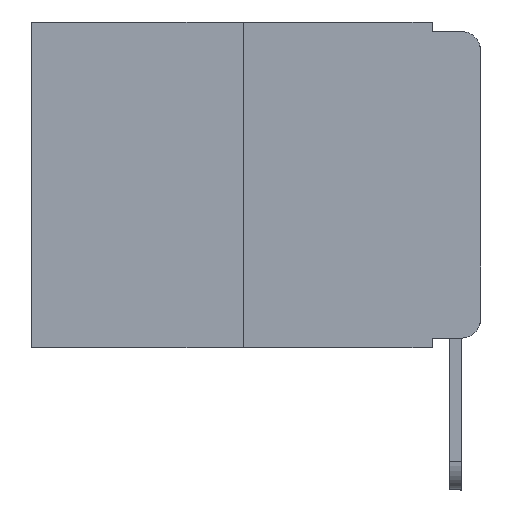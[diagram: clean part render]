
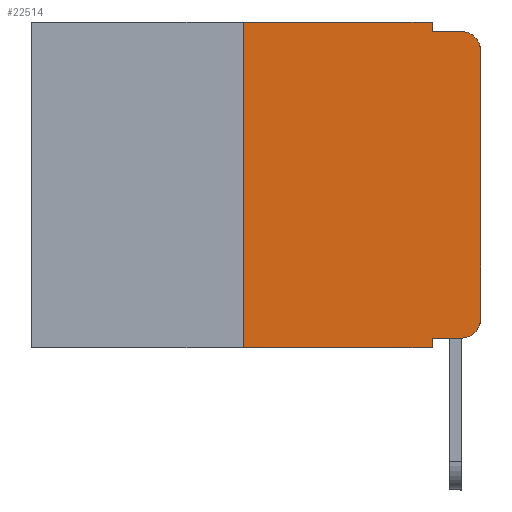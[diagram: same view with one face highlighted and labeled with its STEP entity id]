
A CAD part, left-side view. The second image highlights one B-rep face of the part: STEP entity #22514.
In plain terms, the highlighted planar face has unit normal (-1, 0, 0).
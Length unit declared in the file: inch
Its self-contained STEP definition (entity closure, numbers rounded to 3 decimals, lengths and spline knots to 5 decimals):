
#787 = DIRECTION ( 'NONE',  ( 0., -1., 0. ) ) ;
#1265 = FACE_OUTER_BOUND ( 'NONE', #9231, .T. ) ;
#1446 = CARTESIAN_POINT ( 'NONE',  ( 0., 0.473, -0.343 ) ) ;
#1487 = VECTOR ( 'NONE', #3768, 39.37008 ) ;
#2001 = CARTESIAN_POINT ( 'NONE',  ( 0., 0.051, 0. ) ) ;
#2354 = CARTESIAN_POINT ( 'NONE',  ( 0., 0., 0. ) ) ;
#2392 = LINE ( 'NONE', #24434, #18902 ) ;
#3053 = EDGE_CURVE ( 'NONE', #7344, #7905, #4214, .T. ) ;
#3597 = CIRCLE ( 'NONE', #18939, 0.02 ) ;
#3720 = ORIENTED_EDGE ( 'NONE', *, *, #6366, .T. ) ;
#3768 = DIRECTION ( 'NONE',  ( 0., -1., 0. ) ) ;
#4028 = ORIENTED_EDGE ( 'NONE', *, *, #15728, .F. ) ;
#4088 = EDGE_CURVE ( 'NONE', #20739, #8095, #5442, .T. ) ;
#4214 = LINE ( 'NONE', #2354, #22141 ) ;
#4770 = ORIENTED_EDGE ( 'NONE', *, *, #21895, .T. ) ;
#5196 = DIRECTION ( 'NONE',  ( 0., 0., -1. ) ) ;
#5442 = LINE ( 'NONE', #1446, #24573 ) ;
#5775 = PLANE ( 'NONE',  #18420 ) ;
#5889 = DIRECTION ( 'NONE',  ( 1., 0., 0. ) ) ;
#6028 = DIRECTION ( 'NONE',  ( -1., 0., 0. ) ) ;
#6366 = EDGE_CURVE ( 'NONE', #21354, #7344, #11862, .T. ) ;
#7091 = ORIENTED_EDGE ( 'NONE', *, *, #20962, .F. ) ;
#7268 = CARTESIAN_POINT ( 'NONE',  ( 0., 0.02, -0.01 ) ) ;
#7344 = VERTEX_POINT ( 'NONE', #23245 ) ;
#7723 = ORIENTED_EDGE ( 'NONE', *, *, #14620, .T. ) ;
#7905 = VERTEX_POINT ( 'NONE', #25472 ) ;
#7908 = CARTESIAN_POINT ( 'NONE',  ( 0., 0.051, -0.01 ) ) ;
#7959 = CARTESIAN_POINT ( 'NONE',  ( 0., 0.051, -0.343 ) ) ;
#8036 = CARTESIAN_POINT ( 'NONE',  ( 0., 0.02, -0.313 ) ) ;
#8095 = VERTEX_POINT ( 'NONE', #7959 ) ;
#8491 = VECTOR ( 'NONE', #8730, 39.37008 ) ;
#8730 = DIRECTION ( 'NONE',  ( 0., 0., -1. ) ) ;
#9126 = LINE ( 'NONE', #17406, #21596 ) ;
#9231 = EDGE_LOOP ( 'NONE', ( #17550, #7723, #21815, #7091, #13987, #22833, #19930, #4028, #4770, #3720 ) ) ;
#10171 = AXIS2_PLACEMENT_3D ( 'NONE', #8036, #6028, #15641 ) ;
#10709 = CARTESIAN_POINT ( 'NONE',  ( 0., 0.051, -0.333 ) ) ;
#11021 = VERTEX_POINT ( 'NONE', #23964 ) ;
#11453 = CARTESIAN_POINT ( 'NONE',  ( 0., 0.02, -0.03 ) ) ;
#11862 = CIRCLE ( 'NONE', #10171, 0.02 ) ;
#12736 = DIRECTION ( 'NONE',  ( 0., 0., 1. ) ) ;
#13873 = CARTESIAN_POINT ( 'NONE',  ( 0., 0.25, 0. ) ) ;
#13987 = ORIENTED_EDGE ( 'NONE', *, *, #25727, .F. ) ;
#14620 = EDGE_CURVE ( 'NONE', #7905, #22303, #3597, .T. ) ;
#15067 = LINE ( 'NONE', #16666, #24768 ) ;
#15641 = DIRECTION ( 'NONE',  ( 0., 0., -1. ) ) ;
#15645 = EDGE_CURVE ( 'NONE', #20739, #21565, #9126, .T. ) ;
#15728 = EDGE_CURVE ( 'NONE', #24914, #8095, #16138, .T. ) ;
#16138 = LINE ( 'NONE', #22826, #17756 ) ;
#16666 = CARTESIAN_POINT ( 'NONE',  ( 0., 0.051, -0.333 ) ) ;
#17199 = DIRECTION ( 'NONE',  ( 0., -1., 0. ) ) ;
#17406 = CARTESIAN_POINT ( 'NONE',  ( 0., 0.25, 0. ) ) ;
#17550 = ORIENTED_EDGE ( 'NONE', *, *, #3053, .T. ) ;
#17756 = VECTOR ( 'NONE', #24310, 39.37008 ) ;
#17931 = LINE ( 'NONE', #7908, #1487 ) ;
#18074 = DIRECTION ( 'NONE',  ( 0., 0., -1. ) ) ;
#18420 = AXIS2_PLACEMENT_3D ( 'NONE', #22069, #5889, #18074 ) ;
#18545 = DIRECTION ( 'NONE',  ( 0., -1., 0. ) ) ;
#18902 = VECTOR ( 'NONE', #18545, 39.37008 ) ;
#18939 = AXIS2_PLACEMENT_3D ( 'NONE', #11453, #25780, #5196 ) ;
#19001 = LINE ( 'NONE', #21022, #8491 ) ;
#19714 = CARTESIAN_POINT ( 'NONE',  ( 0., 0.25, -0.343 ) ) ;
#19930 = ORIENTED_EDGE ( 'NONE', *, *, #4088, .T. ) ;
#20590 = CARTESIAN_POINT ( 'NONE',  ( 0., 0.02, -0.333 ) ) ;
#20739 = VERTEX_POINT ( 'NONE', #19714 ) ;
#20962 = EDGE_CURVE ( 'NONE', #24013, #11021, #19001, .T. ) ;
#21022 = CARTESIAN_POINT ( 'NONE',  ( 0., 0.051, 0. ) ) ;
#21354 = VERTEX_POINT ( 'NONE', #20590 ) ;
#21565 = VERTEX_POINT ( 'NONE', #13873 ) ;
#21596 = VECTOR ( 'NONE', #25563, 39.37008 ) ;
#21815 = ORIENTED_EDGE ( 'NONE', *, *, #25170, .F. ) ;
#21895 = EDGE_CURVE ( 'NONE', #24914, #21354, #15067, .T. ) ;
#22069 = CARTESIAN_POINT ( 'NONE',  ( 0., 0.473, 0. ) ) ;
#22141 = VECTOR ( 'NONE', #12736, 39.37008 ) ;
#22303 = VERTEX_POINT ( 'NONE', #7268 ) ;
#22514 = ADVANCED_FACE ( 'NONE', ( #1265 ), #5775, .F. ) ;
#22826 = CARTESIAN_POINT ( 'NONE',  ( 0., 0.051, 0. ) ) ;
#22833 = ORIENTED_EDGE ( 'NONE', *, *, #15645, .F. ) ;
#23245 = CARTESIAN_POINT ( 'NONE',  ( 0., 0., -0.313 ) ) ;
#23964 = CARTESIAN_POINT ( 'NONE',  ( 0., 0.051, -0.01 ) ) ;
#24013 = VERTEX_POINT ( 'NONE', #2001 ) ;
#24310 = DIRECTION ( 'NONE',  ( 0., 0., -1. ) ) ;
#24434 = CARTESIAN_POINT ( 'NONE',  ( 0., 0.473, 0. ) ) ;
#24573 = VECTOR ( 'NONE', #17199, 39.37008 ) ;
#24768 = VECTOR ( 'NONE', #787, 39.37008 ) ;
#24914 = VERTEX_POINT ( 'NONE', #10709 ) ;
#25170 = EDGE_CURVE ( 'NONE', #11021, #22303, #17931, .T. ) ;
#25472 = CARTESIAN_POINT ( 'NONE',  ( 0., 0., -0.03 ) ) ;
#25563 = DIRECTION ( 'NONE',  ( 0., 0., 1. ) ) ;
#25727 = EDGE_CURVE ( 'NONE', #21565, #24013, #2392, .T. ) ;
#25780 = DIRECTION ( 'NONE',  ( -1., 0., 0. ) ) ;
